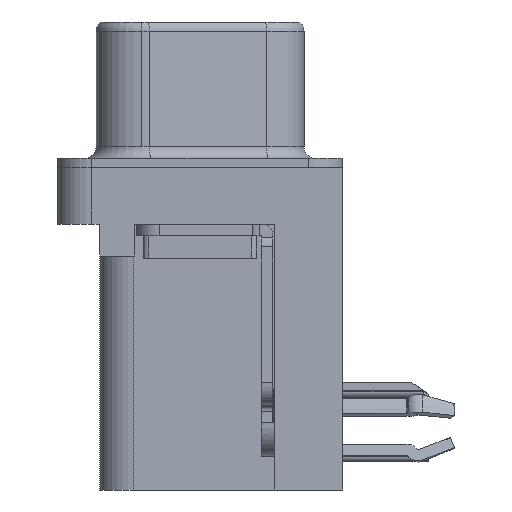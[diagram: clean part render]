
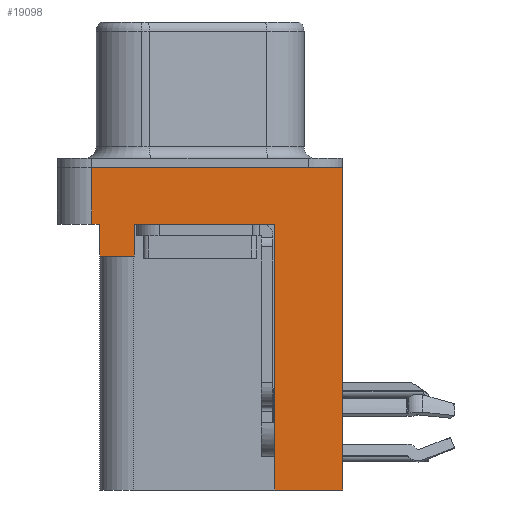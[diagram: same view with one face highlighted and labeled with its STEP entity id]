
A CAD part, left-side view. The second image highlights one B-rep face of the part: STEP entity #19098.
In plain terms, the highlighted planar face has unit normal (-1, 0, 0).
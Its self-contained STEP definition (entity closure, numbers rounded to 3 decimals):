
#288 = VERTEX_POINT ( 'NONE', #18315 ) ;
#1636 = CARTESIAN_POINT ( 'NONE',  ( -3., 4.425, -3.9 ) ) ;
#1688 = EDGE_CURVE ( 'NONE', #15620, #288, #5101, .T. ) ;
#2880 = VECTOR ( 'NONE', #5700, 1000. ) ;
#2948 = DIRECTION ( 'NONE',  ( 0., 1., 0. ) ) ;
#3029 = LINE ( 'NONE', #18242, #21776 ) ;
#3137 = ORIENTED_EDGE ( 'NONE', *, *, #4418, .F. ) ;
#3197 = VERTEX_POINT ( 'NONE', #4125 ) ;
#3471 = VECTOR ( 'NONE', #19890, 1000. ) ;
#3849 = EDGE_CURVE ( 'NONE', #288, #22889, #13266, .T. ) ;
#4125 = CARTESIAN_POINT ( 'NONE',  ( -3., 4.425, -3.9 ) ) ;
#4418 = EDGE_CURVE ( 'NONE', #23322, #12307, #17119, .T. ) ;
#4580 = CARTESIAN_POINT ( 'NONE',  ( -3., -6.275, -2.5 ) ) ;
#4776 = EDGE_LOOP ( 'NONE', ( #7719, #24063, #17698, #14705, #6694, #22599, #7586, #15131, #3137, #8743 ) ) ;
#4836 = CARTESIAN_POINT ( 'NONE',  ( -3., -3.295, -2.5 ) ) ;
#5101 = LINE ( 'NONE', #8622, #8046 ) ;
#5251 = CARTESIAN_POINT ( 'NONE',  ( -3., -3.295, -14.2 ) ) ;
#5448 = VECTOR ( 'NONE', #22728, 1000. ) ;
#5560 = FACE_OUTER_BOUND ( 'NONE', #4776, .T. ) ;
#5611 = VECTOR ( 'NONE', #22848, 1000. ) ;
#5700 = DIRECTION ( 'NONE',  ( 0., 1., 0. ) ) ;
#5850 = EDGE_CURVE ( 'NONE', #12543, #7107, #5947, .T. ) ;
#5947 = LINE ( 'NONE', #13365, #5448 ) ;
#6508 = VECTOR ( 'NONE', #20676, 1000. ) ;
#6694 = ORIENTED_EDGE ( 'NONE', *, *, #11524, .F. ) ;
#6874 = CARTESIAN_POINT ( 'NONE',  ( -3., -6.275, -14.2 ) ) ;
#7107 = VERTEX_POINT ( 'NONE', #15419 ) ;
#7586 = ORIENTED_EDGE ( 'NONE', *, *, #3849, .T. ) ;
#7719 = ORIENTED_EDGE ( 'NONE', *, *, #5850, .F. ) ;
#8046 = VECTOR ( 'NONE', #16061, 1000. ) ;
#8622 = CARTESIAN_POINT ( 'NONE',  ( -3., 2.895, -3.9 ) ) ;
#8743 = ORIENTED_EDGE ( 'NONE', *, *, #15207, .T. ) ;
#9305 = VECTOR ( 'NONE', #23524, 1000. ) ;
#9917 = DIRECTION ( 'NONE',  ( 0., -1., 0. ) ) ;
#10294 = EDGE_CURVE ( 'NONE', #22899, #18897, #21354, .T. ) ;
#10946 = CARTESIAN_POINT ( 'NONE',  ( -3., -6.275, -2.5 ) ) ;
#10981 = AXIS2_PLACEMENT_3D ( 'NONE', #18547, #16859, #24033 ) ;
#11524 = EDGE_CURVE ( 'NONE', #15620, #3197, #22360, .T. ) ;
#12208 = LINE ( 'NONE', #17576, #9305 ) ;
#12307 = VERTEX_POINT ( 'NONE', #5251 ) ;
#12543 = VERTEX_POINT ( 'NONE', #13276 ) ;
#13266 = LINE ( 'NONE', #10946, #6508 ) ;
#13276 = CARTESIAN_POINT ( 'NONE',  ( -3., 4.775, 0. ) ) ;
#13365 = CARTESIAN_POINT ( 'NONE',  ( -3., -6.275, 0. ) ) ;
#13368 = CARTESIAN_POINT ( 'NONE',  ( -3., -3.295, -14.2 ) ) ;
#14448 = CARTESIAN_POINT ( 'NONE',  ( -3., 4.775, -2.5 ) ) ;
#14705 = ORIENTED_EDGE ( 'NONE', *, *, #15301, .F. ) ;
#14916 = PLANE ( 'NONE',  #10981 ) ;
#15131 = ORIENTED_EDGE ( 'NONE', *, *, #21735, .F. ) ;
#15207 = EDGE_CURVE ( 'NONE', #23322, #7107, #12208, .T. ) ;
#15301 = EDGE_CURVE ( 'NONE', #3197, #18897, #16244, .T. ) ;
#15412 = CARTESIAN_POINT ( 'NONE',  ( -3., -3.295, -14.2 ) ) ;
#15419 = CARTESIAN_POINT ( 'NONE',  ( -3., -6.275, 0. ) ) ;
#15420 = LINE ( 'NONE', #13368, #5611 ) ;
#15620 = VERTEX_POINT ( 'NONE', #23270 ) ;
#16061 = DIRECTION ( 'NONE',  ( 0., 0., 1. ) ) ;
#16244 = LINE ( 'NONE', #1636, #3471 ) ;
#16730 = EDGE_CURVE ( 'NONE', #22899, #12543, #3029, .T. ) ;
#16859 = DIRECTION ( 'NONE',  ( -1., 0., 0. ) ) ;
#16874 = VECTOR ( 'NONE', #9917, 1000. ) ;
#17119 = LINE ( 'NONE', #15412, #20139 ) ;
#17576 = CARTESIAN_POINT ( 'NONE',  ( -3., -6.275, -2.5 ) ) ;
#17698 = ORIENTED_EDGE ( 'NONE', *, *, #10294, .T. ) ;
#18242 = CARTESIAN_POINT ( 'NONE',  ( -3., 4.775, -2.5 ) ) ;
#18315 = CARTESIAN_POINT ( 'NONE',  ( -3., 2.895, -2.5 ) ) ;
#18547 = CARTESIAN_POINT ( 'NONE',  ( -3., -6.275, -2.5 ) ) ;
#18897 = VERTEX_POINT ( 'NONE', #19771 ) ;
#19098 = ADVANCED_FACE ( 'NONE', ( #5560 ), #14916, .T. ) ;
#19771 = CARTESIAN_POINT ( 'NONE',  ( -3., 4.425, -2.5 ) ) ;
#19890 = DIRECTION ( 'NONE',  ( 0., 0., 1. ) ) ;
#20139 = VECTOR ( 'NONE', #2948, 1000. ) ;
#20676 = DIRECTION ( 'NONE',  ( 0., -1., 0. ) ) ;
#21354 = LINE ( 'NONE', #4580, #16874 ) ;
#21735 = EDGE_CURVE ( 'NONE', #12307, #22889, #15420, .T. ) ;
#21776 = VECTOR ( 'NONE', #22025, 1000. ) ;
#22025 = DIRECTION ( 'NONE',  ( 0., 0., 1. ) ) ;
#22360 = LINE ( 'NONE', #22482, #2880 ) ;
#22482 = CARTESIAN_POINT ( 'NONE',  ( -3., 4.425, -3.9 ) ) ;
#22599 = ORIENTED_EDGE ( 'NONE', *, *, #1688, .T. ) ;
#22728 = DIRECTION ( 'NONE',  ( 0., -1., 0. ) ) ;
#22848 = DIRECTION ( 'NONE',  ( 0., 0., 1. ) ) ;
#22889 = VERTEX_POINT ( 'NONE', #4836 ) ;
#22899 = VERTEX_POINT ( 'NONE', #14448 ) ;
#23270 = CARTESIAN_POINT ( 'NONE',  ( -3., 2.895, -3.9 ) ) ;
#23322 = VERTEX_POINT ( 'NONE', #6874 ) ;
#23524 = DIRECTION ( 'NONE',  ( 0., 0., 1. ) ) ;
#24033 = DIRECTION ( 'NONE',  ( 0., 0., 1. ) ) ;
#24063 = ORIENTED_EDGE ( 'NONE', *, *, #16730, .F. ) ;
